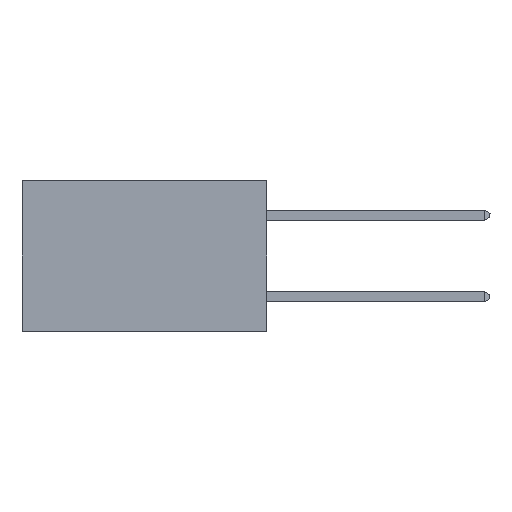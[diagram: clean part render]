
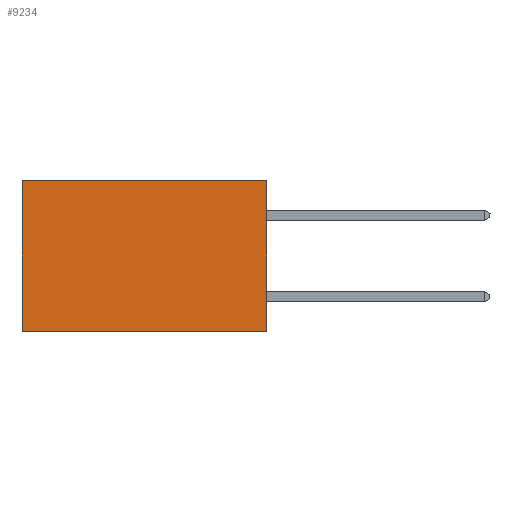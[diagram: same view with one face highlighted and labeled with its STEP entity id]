
A CAD part, left-side view. The second image highlights one B-rep face of the part: STEP entity #9234.
In plain terms, the highlighted planar face has unit normal (-1, 0, 0).
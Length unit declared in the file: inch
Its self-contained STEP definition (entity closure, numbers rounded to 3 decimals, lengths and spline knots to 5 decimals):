
#3161 = ORIENTED_EDGE ( 'NONE', *, *, #17276, .F. ) ;
#3199 = CARTESIAN_POINT ( 'NONE',  ( 0.2875, 0.6, -0.37 ) ) ;
#3327 = LINE ( 'NONE', #11595, #20087 ) ;
#4364 = CARTESIAN_POINT ( 'NONE',  ( 0.2875, 0., 0. ) ) ;
#4851 = AXIS2_PLACEMENT_3D ( 'NONE', #4364, #18919, #17354 ) ;
#5160 = CARTESIAN_POINT ( 'NONE',  ( 0.2875, 0., 0. ) ) ;
#5603 = VECTOR ( 'NONE', #18259, 39.37008 ) ;
#6708 = CARTESIAN_POINT ( 'NONE',  ( 0.2875, 0., -0.37 ) ) ;
#6842 = DIRECTION ( 'NONE',  ( 0., 1., 0. ) ) ;
#7452 = EDGE_LOOP ( 'NONE', ( #19414, #3161, #20353, #17406 ) ) ;
#7843 = EDGE_CURVE ( 'NONE', #9293, #13558, #12970, .T. ) ;
#8118 = VERTEX_POINT ( 'NONE', #5160 ) ;
#8530 = DIRECTION ( 'NONE',  ( 0., 0., -1. ) ) ;
#8984 = VECTOR ( 'NONE', #6842, 39.37008 ) ;
#9234 = ADVANCED_FACE ( 'NONE', ( #16443 ), #18993, .F. ) ;
#9293 = VERTEX_POINT ( 'NONE', #16394 ) ;
#9988 = LINE ( 'NONE', #16814, #8984 ) ;
#11595 = CARTESIAN_POINT ( 'NONE',  ( 0.2875, 0., 0. ) ) ;
#11627 = LINE ( 'NONE', #12946, #19731 ) ;
#12946 = CARTESIAN_POINT ( 'NONE',  ( 0.2875, 0., -0.37 ) ) ;
#12970 = LINE ( 'NONE', #13208, #5603 ) ;
#13208 = CARTESIAN_POINT ( 'NONE',  ( 0.2875, 0.6, 0. ) ) ;
#13558 = VERTEX_POINT ( 'NONE', #3199 ) ;
#13635 = EDGE_CURVE ( 'NONE', #8118, #20333, #3327, .T. ) ;
#16394 = CARTESIAN_POINT ( 'NONE',  ( 0.2875, 0.6, 0. ) ) ;
#16443 = FACE_OUTER_BOUND ( 'NONE', #7452, .T. ) ;
#16814 = CARTESIAN_POINT ( 'NONE',  ( 0.2875, 0., 0. ) ) ;
#17276 = EDGE_CURVE ( 'NONE', #20333, #13558, #11627, .T. ) ;
#17354 = DIRECTION ( 'NONE',  ( 0., 0., -1. ) ) ;
#17406 = ORIENTED_EDGE ( 'NONE', *, *, #19185, .T. ) ;
#18259 = DIRECTION ( 'NONE',  ( 0., 0., -1. ) ) ;
#18919 = DIRECTION ( 'NONE',  ( 1., 0., 0. ) ) ;
#18993 = PLANE ( 'NONE',  #4851 ) ;
#19185 = EDGE_CURVE ( 'NONE', #8118, #9293, #9988, .T. ) ;
#19414 = ORIENTED_EDGE ( 'NONE', *, *, #7843, .T. ) ;
#19731 = VECTOR ( 'NONE', #20941, 39.37008 ) ;
#20087 = VECTOR ( 'NONE', #8530, 39.37008 ) ;
#20333 = VERTEX_POINT ( 'NONE', #6708 ) ;
#20353 = ORIENTED_EDGE ( 'NONE', *, *, #13635, .F. ) ;
#20941 = DIRECTION ( 'NONE',  ( 0., 1., 0. ) ) ;
